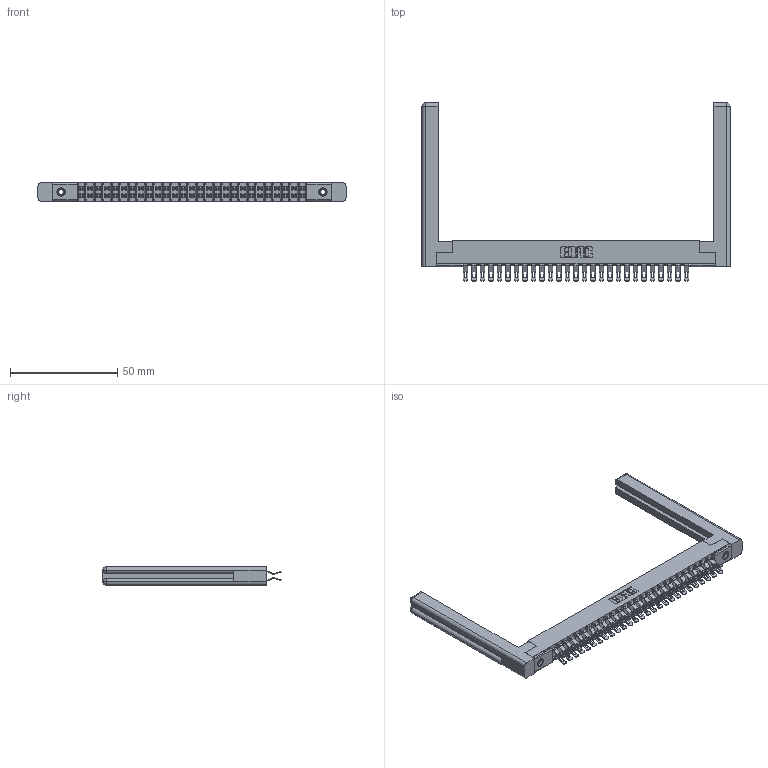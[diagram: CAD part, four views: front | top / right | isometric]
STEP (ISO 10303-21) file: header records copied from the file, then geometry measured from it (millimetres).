
FILE_DESCRIPTION (( 'STEP AP203' ), '1' );
FILE_NAME ('307-054-555-258.STEP', '2019-09-06T13:00:34', ( '' ), ( '' ), 'SwSTEP 2.0', 'SolidWorks 2016', '' );
FILE_SCHEMA (( 'CONFIG_CONTROL_DESIGN' ));
Length unit declared in the file: inch
Products named in the file (5): 307-220-058; 307 Part_.156 Dia Mounting Holes; 345-250-001_345-250-001-102; 307-054-555-258; 307-290-001_555
Assembly tree (59 placements, depth 2):
  307-054-555-258
    307 Part_.156 Dia Mounting Holes
    307-290-001_555  x54
    307-220-058  x2
    345-250-001_345-250-001-102  x2
Bounding box: 143.61 x 83.06 x 8.71 mm (x, y, z)
Volume: 17240.7 mm3; surface area: 23113.6 mm2
Topology: 59 solids, 59 shells, 3582 faces, 10451 edges, 6806 vertices
Faces by surface type: plane 1990, cylinder 1512, sphere 56, torus 12, cone 12
Entity records: 29030 total; most frequent: CARTESIAN_POINT 4778, ORIENTED_EDGE 4678, DIRECTION 4651, EDGE_CURVE 2339, LINE 1773, VECTOR 1773, VERTEX_POINT 1512, AXIS2_PLACEMENT_3D 1439
